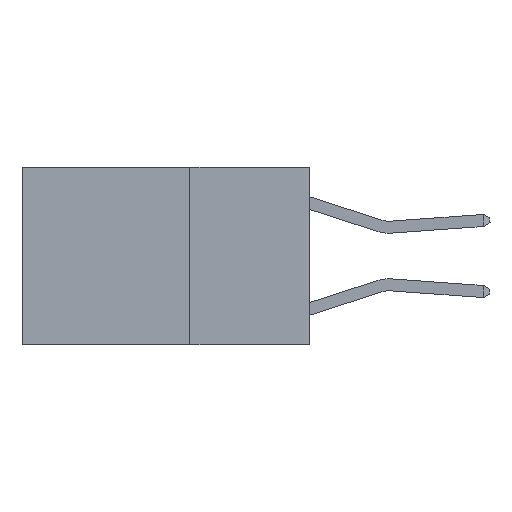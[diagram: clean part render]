
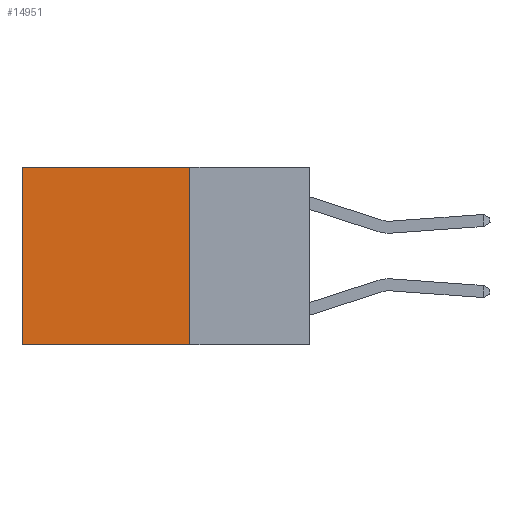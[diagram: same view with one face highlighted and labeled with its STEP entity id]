
A CAD part, left-side view. The second image highlights one B-rep face of the part: STEP entity #14951.
In plain terms, the highlighted planar face has unit normal (-1, 0, 0).
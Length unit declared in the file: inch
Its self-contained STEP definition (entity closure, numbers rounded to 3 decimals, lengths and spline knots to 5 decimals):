
#471 = VERTEX_POINT ( 'NONE', #17841 ) ;
#1278 = EDGE_LOOP ( 'NONE', ( #12831, #2284, #20500, #17002 ) ) ;
#1795 = DIRECTION ( 'NONE',  ( 0., 0., -1. ) ) ;
#2284 = ORIENTED_EDGE ( 'NONE', *, *, #7406, .F. ) ;
#2986 = VECTOR ( 'NONE', #7523, 39.37008 ) ;
#3320 = LINE ( 'NONE', #21387, #3623 ) ;
#3623 = VECTOR ( 'NONE', #23861, 39.37008 ) ;
#4017 = DIRECTION ( 'NONE',  ( 1., 0., 0. ) ) ;
#6680 = VERTEX_POINT ( 'NONE', #16308 ) ;
#6853 = DIRECTION ( 'NONE',  ( 0., 1., 0. ) ) ;
#7081 = EDGE_CURVE ( 'NONE', #6680, #7085, #23128, .T. ) ;
#7085 = VERTEX_POINT ( 'NONE', #9611 ) ;
#7390 = CARTESIAN_POINT ( 'NONE',  ( 0.2625, 0.6, 0. ) ) ;
#7406 = EDGE_CURVE ( 'NONE', #11158, #7085, #20746, .T. ) ;
#7523 = DIRECTION ( 'NONE',  ( 0., 0., -1. ) ) ;
#9455 = VECTOR ( 'NONE', #6853, 39.37008 ) ;
#9611 = CARTESIAN_POINT ( 'NONE',  ( 0.2625, 0.6, -0.37 ) ) ;
#11158 = VERTEX_POINT ( 'NONE', #19384 ) ;
#12642 = EDGE_CURVE ( 'NONE', #471, #6680, #3320, .T. ) ;
#12831 = ORIENTED_EDGE ( 'NONE', *, *, #7081, .T. ) ;
#14605 = VECTOR ( 'NONE', #19025, 39.37008 ) ;
#14951 = ADVANCED_FACE ( 'NONE', ( #19735 ), #21835, .F. ) ;
#16308 = CARTESIAN_POINT ( 'NONE',  ( 0.2625, 0.6, 0. ) ) ;
#16804 = LINE ( 'NONE', #25194, #14605 ) ;
#17002 = ORIENTED_EDGE ( 'NONE', *, *, #12642, .T. ) ;
#17841 = CARTESIAN_POINT ( 'NONE',  ( 0.2625, 0.25, 0. ) ) ;
#17994 = EDGE_CURVE ( 'NONE', #471, #11158, #16804, .T. ) ;
#19025 = DIRECTION ( 'NONE',  ( 0., 0., -1. ) ) ;
#19384 = CARTESIAN_POINT ( 'NONE',  ( 0.2625, 0.25, -0.37 ) ) ;
#19735 = FACE_OUTER_BOUND ( 'NONE', #1278, .T. ) ;
#20500 = ORIENTED_EDGE ( 'NONE', *, *, #17994, .F. ) ;
#20746 = LINE ( 'NONE', #24811, #9455 ) ;
#21387 = CARTESIAN_POINT ( 'NONE',  ( 0.2625, 0.25, 0. ) ) ;
#21835 = PLANE ( 'NONE',  #24563 ) ;
#21958 = CARTESIAN_POINT ( 'NONE',  ( 0.2625, 0.25, 0. ) ) ;
#23128 = LINE ( 'NONE', #7390, #2986 ) ;
#23861 = DIRECTION ( 'NONE',  ( 0., 1., 0. ) ) ;
#24563 = AXIS2_PLACEMENT_3D ( 'NONE', #21958, #4017, #1795 ) ;
#24811 = CARTESIAN_POINT ( 'NONE',  ( 0.2625, 0.25, -0.37 ) ) ;
#25194 = CARTESIAN_POINT ( 'NONE',  ( 0.2625, 0.25, 0. ) ) ;
